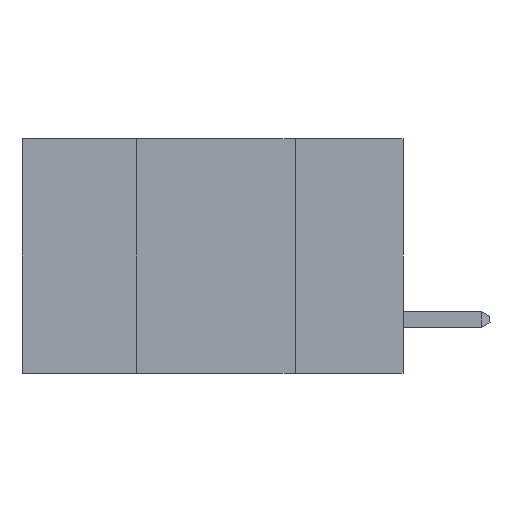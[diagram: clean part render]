
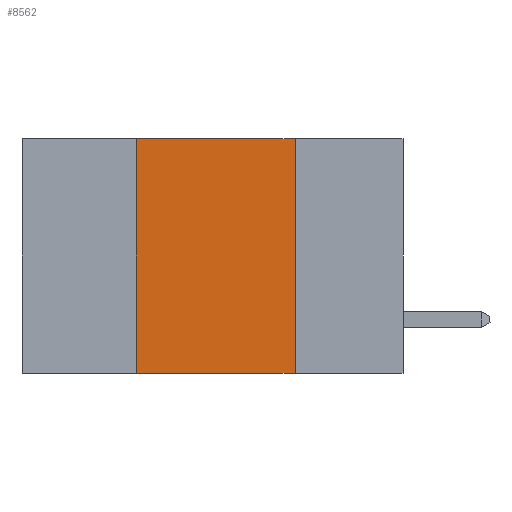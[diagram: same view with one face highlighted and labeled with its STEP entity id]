
A CAD part, left-side view. The second image highlights one B-rep face of the part: STEP entity #8562.
In plain terms, the highlighted planar face has unit normal (-1, 0, 0).
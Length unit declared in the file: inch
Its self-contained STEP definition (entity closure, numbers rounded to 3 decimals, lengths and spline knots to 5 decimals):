
#601 = CARTESIAN_POINT ( 'NONE',  ( 0., 0.6, 0. ) ) ;
#861 = CARTESIAN_POINT ( 'NONE',  ( 0., 0.6, 0. ) ) ;
#1350 = ORIENTED_EDGE ( 'NONE', *, *, #3489, .T. ) ;
#1635 = LINE ( 'NONE', #4092, #4288 ) ;
#1735 = CARTESIAN_POINT ( 'NONE',  ( 0., 0.17, 0. ) ) ;
#1778 = CARTESIAN_POINT ( 'NONE',  ( 0., 0.17, -0.37 ) ) ;
#1785 = DIRECTION ( 'NONE',  ( 0., -1., 0. ) ) ;
#2244 = VERTEX_POINT ( 'NONE', #1778 ) ;
#2487 = VECTOR ( 'NONE', #6764, 39.37008 ) ;
#3489 = EDGE_CURVE ( 'NONE', #7839, #2244, #1635, .T. ) ;
#4092 = CARTESIAN_POINT ( 'NONE',  ( 0., 0.6, -0.37 ) ) ;
#4210 = CARTESIAN_POINT ( 'NONE',  ( 0., 0.42, 0. ) ) ;
#4223 = DIRECTION ( 'NONE',  ( 1., 0., 0. ) ) ;
#4288 = VECTOR ( 'NONE', #8899, 39.37008 ) ;
#5653 = VERTEX_POINT ( 'NONE', #7101 ) ;
#5753 = ORIENTED_EDGE ( 'NONE', *, *, #9820, .F. ) ;
#5962 = FACE_OUTER_BOUND ( 'NONE', #7230, .T. ) ;
#6316 = AXIS2_PLACEMENT_3D ( 'NONE', #601, #4223, #9764 ) ;
#6741 = CARTESIAN_POINT ( 'NONE',  ( 0., 0.42, -0.37 ) ) ;
#6764 = DIRECTION ( 'NONE',  ( 0., 0., 1. ) ) ;
#6996 = LINE ( 'NONE', #4210, #2487 ) ;
#7087 = VECTOR ( 'NONE', #1785, 39.37008 ) ;
#7101 = CARTESIAN_POINT ( 'NONE',  ( 0., 0.42, 0. ) ) ;
#7196 = VECTOR ( 'NONE', #9918, 39.37008 ) ;
#7230 = EDGE_LOOP ( 'NONE', ( #8223, #5753, #7871, #1350 ) ) ;
#7440 = LINE ( 'NONE', #1735, #7196 ) ;
#7839 = VERTEX_POINT ( 'NONE', #6741 ) ;
#7871 = ORIENTED_EDGE ( 'NONE', *, *, #8431, .F. ) ;
#8223 = ORIENTED_EDGE ( 'NONE', *, *, #10381, .F. ) ;
#8431 = EDGE_CURVE ( 'NONE', #7839, #5653, #6996, .T. ) ;
#8562 = ADVANCED_FACE ( 'NONE', ( #5962 ), #9021, .F. ) ;
#8899 = DIRECTION ( 'NONE',  ( 0., -1., 0. ) ) ;
#9021 = PLANE ( 'NONE',  #6316 ) ;
#9364 = LINE ( 'NONE', #861, #7087 ) ;
#9449 = VERTEX_POINT ( 'NONE', #10207 ) ;
#9764 = DIRECTION ( 'NONE',  ( 0., 0., -1. ) ) ;
#9820 = EDGE_CURVE ( 'NONE', #5653, #9449, #9364, .T. ) ;
#9918 = DIRECTION ( 'NONE',  ( 0., 0., -1. ) ) ;
#10207 = CARTESIAN_POINT ( 'NONE',  ( 0., 0.17, 0. ) ) ;
#10381 = EDGE_CURVE ( 'NONE', #9449, #2244, #7440, .T. ) ;
